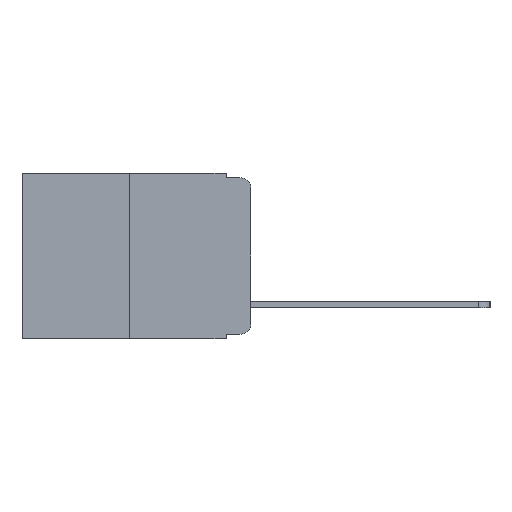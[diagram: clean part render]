
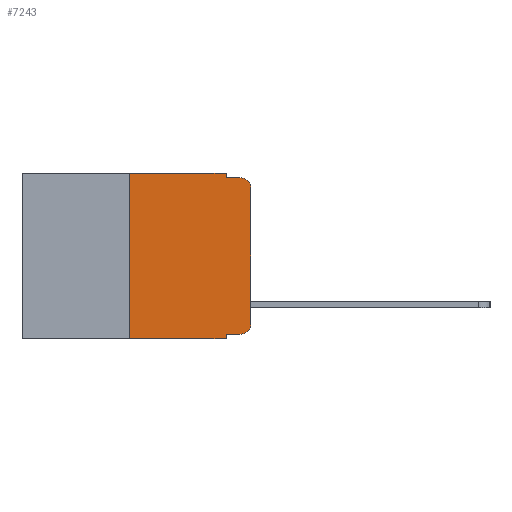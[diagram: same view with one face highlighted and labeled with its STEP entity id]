
A CAD part, left-side view. The second image highlights one B-rep face of the part: STEP entity #7243.
In plain terms, the highlighted planar face has unit normal (-1, 0, 0).
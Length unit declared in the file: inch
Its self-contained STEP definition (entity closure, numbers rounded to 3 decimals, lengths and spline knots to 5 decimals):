
#11 = EDGE_CURVE ( 'NONE', #9297, #1323, #565, .T. ) ;
#359 = ORIENTED_EDGE ( 'NONE', *, *, #2520, .T. ) ;
#565 = LINE ( 'NONE', #6061, #11818 ) ;
#601 = CARTESIAN_POINT ( 'NONE',  ( 0., 0.02, -0.01 ) ) ;
#660 = ORIENTED_EDGE ( 'NONE', *, *, #11, .T. ) ;
#708 = VERTEX_POINT ( 'NONE', #9916 ) ;
#779 = VERTEX_POINT ( 'NONE', #601 ) ;
#1323 = VERTEX_POINT ( 'NONE', #13468 ) ;
#1451 = VECTOR ( 'NONE', #5228, 39.37008 ) ;
#1489 = EDGE_CURVE ( 'NONE', #9297, #10957, #7414, .T. ) ;
#1495 = ORIENTED_EDGE ( 'NONE', *, *, #7182, .F. ) ;
#1666 = ORIENTED_EDGE ( 'NONE', *, *, #1489, .F. ) ;
#1715 = CIRCLE ( 'NONE', #5281, 0.02 ) ;
#1894 = CARTESIAN_POINT ( 'NONE',  ( 0., 0.051, -0.01 ) ) ;
#2232 = EDGE_CURVE ( 'NONE', #11572, #13799, #12844, .T. ) ;
#2420 = DIRECTION ( 'NONE',  ( 0., -1., 0. ) ) ;
#2520 = EDGE_CURVE ( 'NONE', #12875, #11275, #10361, .T. ) ;
#2660 = VECTOR ( 'NONE', #2420, 39.37008 ) ;
#2767 = VECTOR ( 'NONE', #11769, 39.37008 ) ;
#2889 = ORIENTED_EDGE ( 'NONE', *, *, #4846, .T. ) ;
#2946 = DIRECTION ( 'NONE',  ( 1., 0., 0. ) ) ;
#3016 = EDGE_CURVE ( 'NONE', #13799, #779, #11273, .T. ) ;
#3102 = CARTESIAN_POINT ( 'NONE',  ( 0., 0.02, -0.313 ) ) ;
#3148 = DIRECTION ( 'NONE',  ( 0., -1., 0. ) ) ;
#3150 = DIRECTION ( 'NONE',  ( 0., 0., -1. ) ) ;
#3933 = VECTOR ( 'NONE', #7206, 39.37008 ) ;
#4846 = EDGE_CURVE ( 'NONE', #9976, #12875, #11684, .T. ) ;
#5086 = VECTOR ( 'NONE', #11307, 39.37008 ) ;
#5145 = CARTESIAN_POINT ( 'NONE',  ( 0., 0.051, 0. ) ) ;
#5160 = ORIENTED_EDGE ( 'NONE', *, *, #7651, .T. ) ;
#5228 = DIRECTION ( 'NONE',  ( 0., 0., -1. ) ) ;
#5276 = ORIENTED_EDGE ( 'NONE', *, *, #5347, .T. ) ;
#5281 = AXIS2_PLACEMENT_3D ( 'NONE', #13737, #12802, #12773 ) ;
#5347 = EDGE_CURVE ( 'NONE', #708, #779, #1715, .T. ) ;
#5615 = LINE ( 'NONE', #6291, #13492 ) ;
#6061 = CARTESIAN_POINT ( 'NONE',  ( 0., 0.473, -0.343 ) ) ;
#6291 = CARTESIAN_POINT ( 'NONE',  ( 0., 0., 0. ) ) ;
#6616 = CARTESIAN_POINT ( 'NONE',  ( 0., 0.051, -0.01 ) ) ;
#6684 = CARTESIAN_POINT ( 'NONE',  ( 0., 0.25, 0. ) ) ;
#6743 = CARTESIAN_POINT ( 'NONE',  ( 0., 0.051, 0. ) ) ;
#6792 = EDGE_LOOP ( 'NONE', ( #5160, #5276, #7378, #7310, #7010, #1666, #660, #1495, #2889, #359 ) ) ;
#7010 = ORIENTED_EDGE ( 'NONE', *, *, #13019, .F. ) ;
#7182 = EDGE_CURVE ( 'NONE', #9976, #1323, #10713, .T. ) ;
#7206 = DIRECTION ( 'NONE',  ( 0., 0., 1. ) ) ;
#7243 = ADVANCED_FACE ( 'NONE', ( #9172 ), #13485, .F. ) ;
#7310 = ORIENTED_EDGE ( 'NONE', *, *, #2232, .F. ) ;
#7378 = ORIENTED_EDGE ( 'NONE', *, *, #3016, .F. ) ;
#7414 = LINE ( 'NONE', #11629, #3933 ) ;
#7447 = DIRECTION ( 'NONE',  ( 0., 0., 1. ) ) ;
#7551 = CARTESIAN_POINT ( 'NONE',  ( 0., 0.02, -0.333 ) ) ;
#7651 = EDGE_CURVE ( 'NONE', #11275, #708, #5615, .T. ) ;
#8456 = CARTESIAN_POINT ( 'NONE',  ( 0., 0., -0.313 ) ) ;
#8746 = CARTESIAN_POINT ( 'NONE',  ( 0., 0.25, -0.343 ) ) ;
#9172 = FACE_OUTER_BOUND ( 'NONE', #6792, .T. ) ;
#9297 = VERTEX_POINT ( 'NONE', #8746 ) ;
#9497 = VECTOR ( 'NONE', #3148, 39.37008 ) ;
#9553 = CARTESIAN_POINT ( 'NONE',  ( 0., 0.473, 0. ) ) ;
#9635 = AXIS2_PLACEMENT_3D ( 'NONE', #3102, #12002, #3150 ) ;
#9916 = CARTESIAN_POINT ( 'NONE',  ( 0., 0., -0.03 ) ) ;
#9976 = VERTEX_POINT ( 'NONE', #10542 ) ;
#10326 = CARTESIAN_POINT ( 'NONE',  ( 0., 0.051, 0. ) ) ;
#10361 = CIRCLE ( 'NONE', #9635, 0.02 ) ;
#10463 = AXIS2_PLACEMENT_3D ( 'NONE', #9553, #2946, #10533 ) ;
#10533 = DIRECTION ( 'NONE',  ( 0., 0., -1. ) ) ;
#10542 = CARTESIAN_POINT ( 'NONE',  ( 0., 0.051, -0.333 ) ) ;
#10678 = CARTESIAN_POINT ( 'NONE',  ( 0., 0.473, 0. ) ) ;
#10713 = LINE ( 'NONE', #10326, #5086 ) ;
#10957 = VERTEX_POINT ( 'NONE', #6684 ) ;
#11273 = LINE ( 'NONE', #6616, #2660 ) ;
#11275 = VERTEX_POINT ( 'NONE', #8456 ) ;
#11307 = DIRECTION ( 'NONE',  ( 0., 0., -1. ) ) ;
#11572 = VERTEX_POINT ( 'NONE', #6743 ) ;
#11629 = CARTESIAN_POINT ( 'NONE',  ( 0., 0.25, 0. ) ) ;
#11684 = LINE ( 'NONE', #12952, #2767 ) ;
#11769 = DIRECTION ( 'NONE',  ( 0., -1., 0. ) ) ;
#11818 = VECTOR ( 'NONE', #12054, 39.37008 ) ;
#12002 = DIRECTION ( 'NONE',  ( -1., 0., 0. ) ) ;
#12054 = DIRECTION ( 'NONE',  ( 0., -1., 0. ) ) ;
#12121 = LINE ( 'NONE', #10678, #9497 ) ;
#12773 = DIRECTION ( 'NONE',  ( 0., 0., -1. ) ) ;
#12802 = DIRECTION ( 'NONE',  ( -1., 0., 0. ) ) ;
#12844 = LINE ( 'NONE', #5145, #1451 ) ;
#12875 = VERTEX_POINT ( 'NONE', #7551 ) ;
#12952 = CARTESIAN_POINT ( 'NONE',  ( 0., 0.051, -0.333 ) ) ;
#13019 = EDGE_CURVE ( 'NONE', #10957, #11572, #12121, .T. ) ;
#13468 = CARTESIAN_POINT ( 'NONE',  ( 0., 0.051, -0.343 ) ) ;
#13485 = PLANE ( 'NONE',  #10463 ) ;
#13492 = VECTOR ( 'NONE', #7447, 39.37008 ) ;
#13737 = CARTESIAN_POINT ( 'NONE',  ( 0., 0.02, -0.03 ) ) ;
#13799 = VERTEX_POINT ( 'NONE', #1894 ) ;
